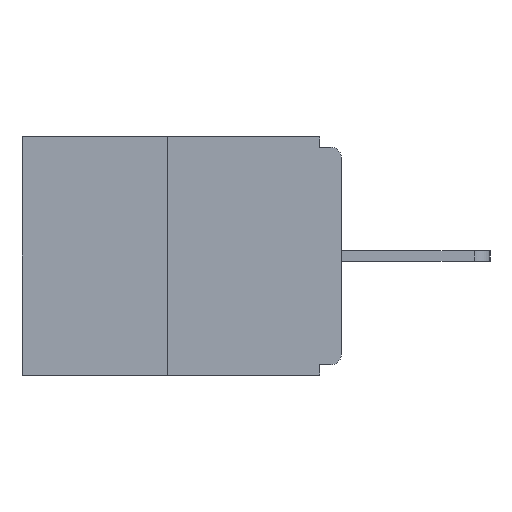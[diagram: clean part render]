
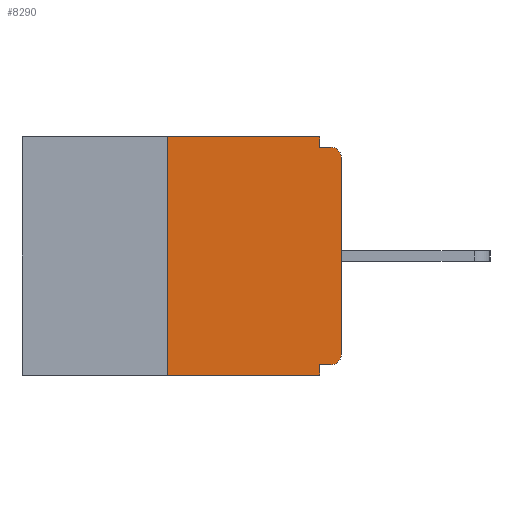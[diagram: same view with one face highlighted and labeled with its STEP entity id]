
A CAD part, left-side view. The second image highlights one B-rep face of the part: STEP entity #8290.
In plain terms, the highlighted planar face has unit normal (-1, 0, 0).
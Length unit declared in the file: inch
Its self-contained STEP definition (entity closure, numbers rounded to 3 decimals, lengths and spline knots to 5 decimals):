
#205 = LINE ( 'NONE', #12160, #9525 ) ;
#214 = CARTESIAN_POINT ( 'NONE',  ( 0., 0., 0. ) ) ;
#381 = ORIENTED_EDGE ( 'NONE', *, *, #12682, .F. ) ;
#725 = CARTESIAN_POINT ( 'NONE',  ( 0., 0., -0.313 ) ) ;
#931 = CARTESIAN_POINT ( 'NONE',  ( 0., 0.031, 0. ) ) ;
#975 = LINE ( 'NONE', #11386, #7129 ) ;
#1692 = CARTESIAN_POINT ( 'NONE',  ( 0., 0.46, 0. ) ) ;
#2077 = ORIENTED_EDGE ( 'NONE', *, *, #10942, .F. ) ;
#2151 = VERTEX_POINT ( 'NONE', #8459 ) ;
#2168 = CARTESIAN_POINT ( 'NONE',  ( 0., 0.25, 0. ) ) ;
#2400 = CARTESIAN_POINT ( 'NONE',  ( 0., 0.25, -0.343 ) ) ;
#2547 = VERTEX_POINT ( 'NONE', #3051 ) ;
#2883 = CARTESIAN_POINT ( 'NONE',  ( 0., 0.25, 0. ) ) ;
#3043 = EDGE_CURVE ( 'NONE', #2151, #3360, #10301, .T. ) ;
#3051 = CARTESIAN_POINT ( 'NONE',  ( 0., 0.015, -0.015 ) ) ;
#3176 = DIRECTION ( 'NONE',  ( 0., 0., -1. ) ) ;
#3360 = VERTEX_POINT ( 'NONE', #3923 ) ;
#3688 = ORIENTED_EDGE ( 'NONE', *, *, #11322, .F. ) ;
#3792 = AXIS2_PLACEMENT_3D ( 'NONE', #9747, #14075, #7470 ) ;
#3923 = CARTESIAN_POINT ( 'NONE',  ( 0., 0.031, -0.328 ) ) ;
#4213 = CARTESIAN_POINT ( 'NONE',  ( 0., 0.46, -0.343 ) ) ;
#4302 = DIRECTION ( 'NONE',  ( -1., 0., 0. ) ) ;
#4491 = VERTEX_POINT ( 'NONE', #12157 ) ;
#4937 = LINE ( 'NONE', #214, #10802 ) ;
#5799 = LINE ( 'NONE', #931, #14083 ) ;
#5814 = EDGE_CURVE ( 'NONE', #12822, #2547, #10536, .T. ) ;
#5863 = DIRECTION ( 'NONE',  ( 0., 0., -1. ) ) ;
#5947 = LINE ( 'NONE', #4213, #8821 ) ;
#6122 = ORIENTED_EDGE ( 'NONE', *, *, #9091, .T. ) ;
#6313 = DIRECTION ( 'NONE',  ( 0., 0., 1. ) ) ;
#6365 = VECTOR ( 'NONE', #12246, 39.37008 ) ;
#6621 = FACE_OUTER_BOUND ( 'NONE', #8974, .T. ) ;
#6808 = AXIS2_PLACEMENT_3D ( 'NONE', #9012, #8965, #8944 ) ;
#7129 = VECTOR ( 'NONE', #3176, 39.37008 ) ;
#7219 = VECTOR ( 'NONE', #11523, 39.37008 ) ;
#7470 = DIRECTION ( 'NONE',  ( 0., 0., -1. ) ) ;
#8052 = CARTESIAN_POINT ( 'NONE',  ( 0., 0.031, -0.015 ) ) ;
#8134 = AXIS2_PLACEMENT_3D ( 'NONE', #11275, #4302, #12355 ) ;
#8290 = ADVANCED_FACE ( 'NONE', ( #6621 ), #13007, .F. ) ;
#8459 = CARTESIAN_POINT ( 'NONE',  ( 0., 0.015, -0.328 ) ) ;
#8763 = LINE ( 'NONE', #2168, #11289 ) ;
#8799 = EDGE_CURVE ( 'NONE', #13828, #12822, #4937, .T. ) ;
#8821 = VECTOR ( 'NONE', #12265, 39.37008 ) ;
#8944 = DIRECTION ( 'NONE',  ( 0., 0., -1. ) ) ;
#8965 = DIRECTION ( 'NONE',  ( -1., 0., 0. ) ) ;
#8974 = EDGE_LOOP ( 'NONE', ( #2077, #11505, #14385, #8995, #11825, #6122, #9348, #9674, #381, #3688 ) ) ;
#8995 = ORIENTED_EDGE ( 'NONE', *, *, #12009, .F. ) ;
#9012 = CARTESIAN_POINT ( 'NONE',  ( 0., 0.015, -0.03 ) ) ;
#9089 = CARTESIAN_POINT ( 'NONE',  ( 0., 0., -0.03 ) ) ;
#9091 = EDGE_CURVE ( 'NONE', #2151, #13828, #13808, .T. ) ;
#9348 = ORIENTED_EDGE ( 'NONE', *, *, #8799, .T. ) ;
#9525 = VECTOR ( 'NONE', #11113, 39.37008 ) ;
#9566 = LINE ( 'NONE', #1692, #6365 ) ;
#9674 = ORIENTED_EDGE ( 'NONE', *, *, #5814, .T. ) ;
#9747 = CARTESIAN_POINT ( 'NONE',  ( 0., 0.46, 0. ) ) ;
#10301 = LINE ( 'NONE', #11285, #7219 ) ;
#10536 = CIRCLE ( 'NONE', #6808, 0.015 ) ;
#10802 = VECTOR ( 'NONE', #6313, 39.37008 ) ;
#10942 = EDGE_CURVE ( 'NONE', #14607, #12368, #9566, .T. ) ;
#11087 = VERTEX_POINT ( 'NONE', #8052 ) ;
#11113 = DIRECTION ( 'NONE',  ( 0., -1., 0. ) ) ;
#11275 = CARTESIAN_POINT ( 'NONE',  ( 0., 0.015, -0.313 ) ) ;
#11285 = CARTESIAN_POINT ( 'NONE',  ( 0., 0., -0.328 ) ) ;
#11289 = VECTOR ( 'NONE', #12699, 39.37008 ) ;
#11322 = EDGE_CURVE ( 'NONE', #12368, #11087, #5799, .T. ) ;
#11386 = CARTESIAN_POINT ( 'NONE',  ( 0., 0.031, -0.343 ) ) ;
#11505 = ORIENTED_EDGE ( 'NONE', *, *, #14932, .F. ) ;
#11523 = DIRECTION ( 'NONE',  ( 0., 1., 0. ) ) ;
#11825 = ORIENTED_EDGE ( 'NONE', *, *, #3043, .F. ) ;
#12009 = EDGE_CURVE ( 'NONE', #3360, #4491, #975, .T. ) ;
#12157 = CARTESIAN_POINT ( 'NONE',  ( 0., 0.031, -0.343 ) ) ;
#12160 = CARTESIAN_POINT ( 'NONE',  ( 0., 0., -0.015 ) ) ;
#12246 = DIRECTION ( 'NONE',  ( 0., -1., 0. ) ) ;
#12265 = DIRECTION ( 'NONE',  ( 0., -1., 0. ) ) ;
#12355 = DIRECTION ( 'NONE',  ( 0., 0., -1. ) ) ;
#12368 = VERTEX_POINT ( 'NONE', #15012 ) ;
#12386 = VERTEX_POINT ( 'NONE', #2400 ) ;
#12682 = EDGE_CURVE ( 'NONE', #11087, #2547, #205, .T. ) ;
#12699 = DIRECTION ( 'NONE',  ( 0., 0., 1. ) ) ;
#12772 = EDGE_CURVE ( 'NONE', #12386, #4491, #5947, .T. ) ;
#12822 = VERTEX_POINT ( 'NONE', #9089 ) ;
#13007 = PLANE ( 'NONE',  #3792 ) ;
#13808 = CIRCLE ( 'NONE', #8134, 0.015 ) ;
#13828 = VERTEX_POINT ( 'NONE', #725 ) ;
#14075 = DIRECTION ( 'NONE',  ( 1., 0., 0. ) ) ;
#14083 = VECTOR ( 'NONE', #5863, 39.37008 ) ;
#14385 = ORIENTED_EDGE ( 'NONE', *, *, #12772, .T. ) ;
#14607 = VERTEX_POINT ( 'NONE', #2883 ) ;
#14932 = EDGE_CURVE ( 'NONE', #12386, #14607, #8763, .T. ) ;
#15012 = CARTESIAN_POINT ( 'NONE',  ( 0., 0.031, 0. ) ) ;
